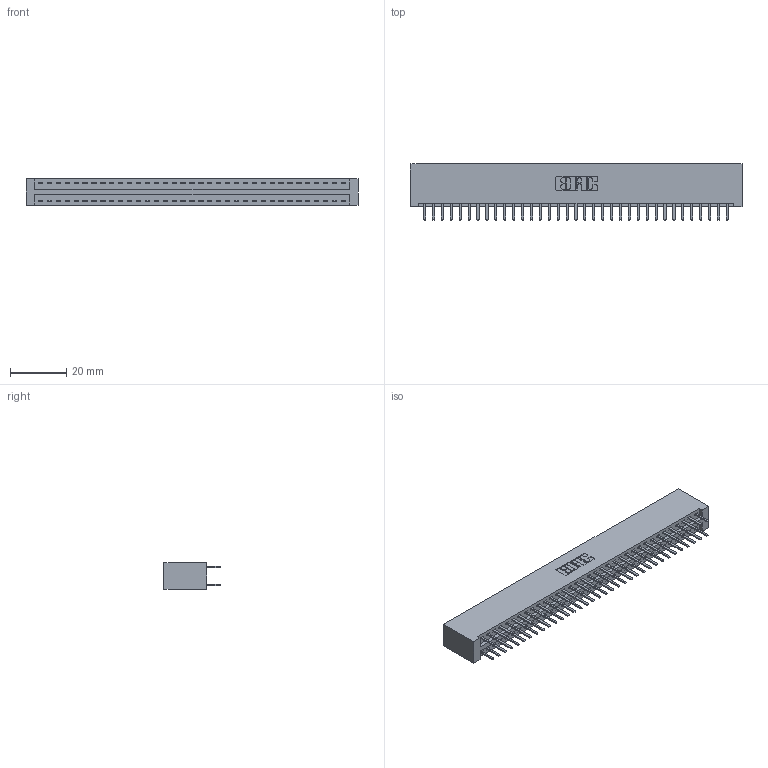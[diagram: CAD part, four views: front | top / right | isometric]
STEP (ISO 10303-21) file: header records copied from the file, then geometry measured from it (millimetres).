
FILE_DESCRIPTION (( 'STEP AP203' ), '1' );
FILE_NAME ('346-070-520-201.STEP', '2018-08-28T22:50:02', ( '' ), ( '' ), 'SwSTEP 2.0', 'SolidWorks 2016', '' );
FILE_SCHEMA (( 'CONFIG_CONTROL_DESIGN' ));
Length unit declared in the file: inch
Products named in the file (3): 346 Part_No Mounting Lugs; 345-292-001_345-293-120; 346-070-520-201
Assembly tree (71 placements, depth 2):
  346-070-520-201
    346 Part_No Mounting Lugs
    345-292-001_345-293-120  x70
Bounding box: 118.36 x 20.02 x 9.4 mm (x, y, z)
Volume: 12030.1 mm3; surface area: 16517.2 mm2
Topology: 71 solids, 71 shells, 4034 faces, 11715 edges, 7622 vertices
Faces by surface type: plane 2662, cylinder 1372
Entity records: 23621 total; most frequent: CARTESIAN_POINT 3912, ORIENTED_EDGE 3834, DIRECTION 3481, EDGE_CURVE 1917, VECTOR 1649, LINE 1649, VERTEX_POINT 1274, AXIS2_PLACEMENT_3D 916
